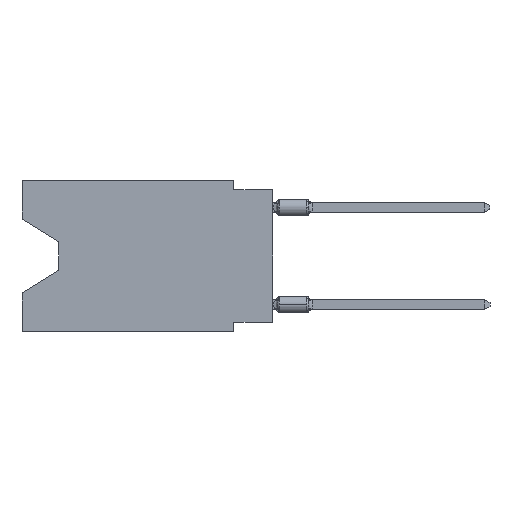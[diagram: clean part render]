
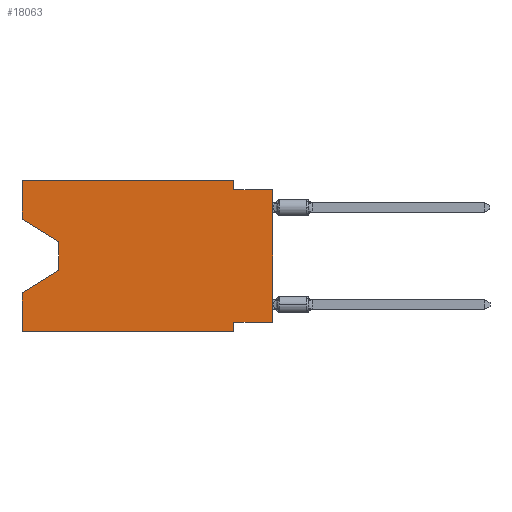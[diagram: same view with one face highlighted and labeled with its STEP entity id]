
A CAD part, left-side view. The second image highlights one B-rep face of the part: STEP entity #18063.
In plain terms, the highlighted planar face has unit normal (-1, 0, 0).
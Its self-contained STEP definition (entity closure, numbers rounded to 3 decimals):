
#733 = EDGE_LOOP ( 'NONE', ( #16544, #21899, #18236, #22593, #3732, #11475, #11462, #2564, #8232, #22380, #11985, #18696 ) ) ;
#1851 = EDGE_CURVE ( 'NONE', #11920, #8776, #15945, .T. ) ;
#1892 = EDGE_CURVE ( 'NONE', #4138, #22835, #19355, .T. ) ;
#2327 = CARTESIAN_POINT ( 'NONE',  ( 0., 16.383, -7.36 ) ) ;
#2465 = LINE ( 'NONE', #6099, #15036 ) ;
#2564 = ORIENTED_EDGE ( 'NONE', *, *, #6916, .T. ) ;
#3732 = ORIENTED_EDGE ( 'NONE', *, *, #15991, .T. ) ;
#3756 = CARTESIAN_POINT ( 'NONE',  ( 0., 2.54, -9.906 ) ) ;
#3963 = CARTESIAN_POINT ( 'NONE',  ( 0., 2.54, -9.271 ) ) ;
#3972 = CARTESIAN_POINT ( 'NONE',  ( 0., 13.97, -4.013 ) ) ;
#4138 = VERTEX_POINT ( 'NONE', #25060 ) ;
#4173 = DIRECTION ( 'NONE',  ( 0., -1., 0. ) ) ;
#4194 = CARTESIAN_POINT ( 'NONE',  ( 0., 13.97, -5.893 ) ) ;
#4333 = VERTEX_POINT ( 'NONE', #3963 ) ;
#4337 = VECTOR ( 'NONE', #10142, 1000. ) ;
#4355 = VECTOR ( 'NONE', #5643, 1000. ) ;
#5509 = CARTESIAN_POINT ( 'NONE',  ( 0., 2.54, -9.906 ) ) ;
#5643 = DIRECTION ( 'NONE',  ( 0., 0., -1. ) ) ;
#5751 = LINE ( 'NONE', #4194, #4337 ) ;
#5783 = CARTESIAN_POINT ( 'NONE',  ( 0., 2.54, 0. ) ) ;
#6052 = VECTOR ( 'NONE', #12988, 1000. ) ;
#6099 = CARTESIAN_POINT ( 'NONE',  ( 0., 0., 0. ) ) ;
#6504 = VECTOR ( 'NONE', #21025, 1000. ) ;
#6916 = EDGE_CURVE ( 'NONE', #12469, #11215, #2465, .T. ) ;
#7034 = CARTESIAN_POINT ( 'NONE',  ( 0., 16.383, -9.906 ) ) ;
#7920 = LINE ( 'NONE', #23712, #11935 ) ;
#8112 = CARTESIAN_POINT ( 'NONE',  ( 0., 16.383, 0. ) ) ;
#8117 = EDGE_CURVE ( 'NONE', #18733, #13776, #5751, .T. ) ;
#8232 = ORIENTED_EDGE ( 'NONE', *, *, #18684, .F. ) ;
#8310 = LINE ( 'NONE', #14386, #24133 ) ;
#8776 = VERTEX_POINT ( 'NONE', #11339 ) ;
#8787 = EDGE_CURVE ( 'NONE', #4333, #25450, #19366, .T. ) ;
#9502 = VECTOR ( 'NONE', #19738, 1000. ) ;
#10065 = EDGE_CURVE ( 'NONE', #4138, #11920, #14179, .T. ) ;
#10142 = DIRECTION ( 'NONE',  ( 0., 0.855, -0.519 ) ) ;
#10448 = CARTESIAN_POINT ( 'NONE',  ( 0., 13.97, -4.013 ) ) ;
#11075 = CARTESIAN_POINT ( 'NONE',  ( 0., 16.383, 0. ) ) ;
#11215 = VERTEX_POINT ( 'NONE', #16246 ) ;
#11239 = VECTOR ( 'NONE', #21942, 1000. ) ;
#11339 = CARTESIAN_POINT ( 'NONE',  ( 0., 2.54, 0. ) ) ;
#11462 = ORIENTED_EDGE ( 'NONE', *, *, #25068, .F. ) ;
#11475 = ORIENTED_EDGE ( 'NONE', *, *, #8787, .F. ) ;
#11482 = CARTESIAN_POINT ( 'NONE',  ( 0., 16.383, -9.906 ) ) ;
#11714 = EDGE_CURVE ( 'NONE', #22694, #13776, #23875, .T. ) ;
#11920 = VERTEX_POINT ( 'NONE', #24374 ) ;
#11935 = VECTOR ( 'NONE', #25535, 1000. ) ;
#11985 = ORIENTED_EDGE ( 'NONE', *, *, #1851, .F. ) ;
#12469 = VERTEX_POINT ( 'NONE', #16252 ) ;
#12988 = DIRECTION ( 'NONE',  ( 0., -1., 0. ) ) ;
#13018 = FACE_OUTER_BOUND ( 'NONE', #733, .T. ) ;
#13397 = CARTESIAN_POINT ( 'NONE',  ( 0., 16.383, 0. ) ) ;
#13776 = VERTEX_POINT ( 'NONE', #2327 ) ;
#14179 = LINE ( 'NONE', #8112, #11239 ) ;
#14200 = CARTESIAN_POINT ( 'NONE',  ( 0., 2.54, -0.635 ) ) ;
#14386 = CARTESIAN_POINT ( 'NONE',  ( 0., 0., -0.635 ) ) ;
#14966 = VECTOR ( 'NONE', #25466, 1000. ) ;
#15036 = VECTOR ( 'NONE', #20196, 1000. ) ;
#15100 = LINE ( 'NONE', #5783, #14966 ) ;
#15215 = DIRECTION ( 'NONE',  ( 0., 0., -1. ) ) ;
#15945 = LINE ( 'NONE', #13397, #18080 ) ;
#15991 = EDGE_CURVE ( 'NONE', #22694, #25450, #24767, .T. ) ;
#16067 = VECTOR ( 'NONE', #16276, 1000. ) ;
#16246 = CARTESIAN_POINT ( 'NONE',  ( 0., 0., -0.635 ) ) ;
#16252 = CARTESIAN_POINT ( 'NONE',  ( 0., 0., -9.271 ) ) ;
#16276 = DIRECTION ( 'NONE',  ( 0., 0., -1. ) ) ;
#16544 = ORIENTED_EDGE ( 'NONE', *, *, #1892, .T. ) ;
#17758 = CARTESIAN_POINT ( 'NONE',  ( 0., 16.383, -2.546 ) ) ;
#17913 = CARTESIAN_POINT ( 'NONE',  ( 0., 16.383, 0. ) ) ;
#18063 = ADVANCED_FACE ( 'NONE', ( #13018 ), #20909, .F. ) ;
#18080 = VECTOR ( 'NONE', #4173, 1000. ) ;
#18218 = LINE ( 'NONE', #10448, #16067 ) ;
#18236 = ORIENTED_EDGE ( 'NONE', *, *, #8117, .T. ) ;
#18684 = EDGE_CURVE ( 'NONE', #21118, #11215, #8310, .T. ) ;
#18696 = ORIENTED_EDGE ( 'NONE', *, *, #10065, .F. ) ;
#18733 = VERTEX_POINT ( 'NONE', #24351 ) ;
#18837 = DIRECTION ( 'NONE',  ( 1., 0., 0. ) ) ;
#19355 = LINE ( 'NONE', #17758, #6504 ) ;
#19366 = LINE ( 'NONE', #5509, #4355 ) ;
#19738 = DIRECTION ( 'NONE',  ( 0., 0., 1. ) ) ;
#20196 = DIRECTION ( 'NONE',  ( 0., 0., 1. ) ) ;
#20909 = PLANE ( 'NONE',  #23707 ) ;
#21025 = DIRECTION ( 'NONE',  ( 0., -0.855, -0.519 ) ) ;
#21118 = VERTEX_POINT ( 'NONE', #14200 ) ;
#21899 = ORIENTED_EDGE ( 'NONE', *, *, #25585, .T. ) ;
#21942 = DIRECTION ( 'NONE',  ( 0., 0., 1. ) ) ;
#22280 = DIRECTION ( 'NONE',  ( 0., -1., 0. ) ) ;
#22380 = ORIENTED_EDGE ( 'NONE', *, *, #24011, .F. ) ;
#22593 = ORIENTED_EDGE ( 'NONE', *, *, #11714, .F. ) ;
#22694 = VERTEX_POINT ( 'NONE', #11482 ) ;
#22835 = VERTEX_POINT ( 'NONE', #3972 ) ;
#23707 = AXIS2_PLACEMENT_3D ( 'NONE', #11075, #18837, #15215 ) ;
#23712 = CARTESIAN_POINT ( 'NONE',  ( 0., 0., -9.271 ) ) ;
#23875 = LINE ( 'NONE', #17913, #9502 ) ;
#24011 = EDGE_CURVE ( 'NONE', #8776, #21118, #15100, .T. ) ;
#24133 = VECTOR ( 'NONE', #22280, 1000. ) ;
#24351 = CARTESIAN_POINT ( 'NONE',  ( 0., 13.97, -5.893 ) ) ;
#24374 = CARTESIAN_POINT ( 'NONE',  ( 0., 16.383, 0. ) ) ;
#24767 = LINE ( 'NONE', #7034, #6052 ) ;
#25060 = CARTESIAN_POINT ( 'NONE',  ( 0., 16.383, -2.546 ) ) ;
#25068 = EDGE_CURVE ( 'NONE', #12469, #4333, #7920, .T. ) ;
#25450 = VERTEX_POINT ( 'NONE', #3756 ) ;
#25466 = DIRECTION ( 'NONE',  ( 0., 0., -1. ) ) ;
#25535 = DIRECTION ( 'NONE',  ( 0., 1., 0. ) ) ;
#25585 = EDGE_CURVE ( 'NONE', #22835, #18733, #18218, .T. ) ;
